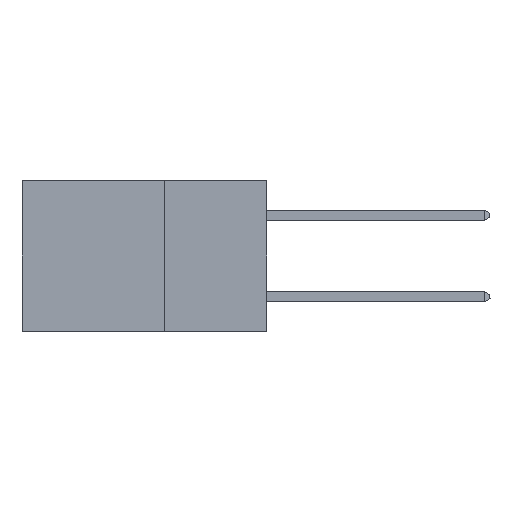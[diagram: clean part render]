
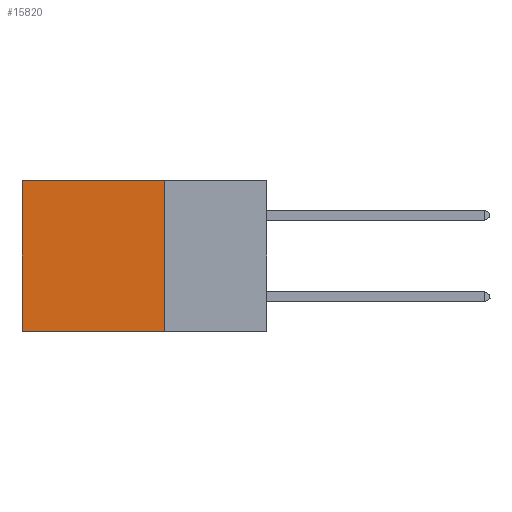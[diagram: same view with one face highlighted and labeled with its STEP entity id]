
A CAD part, left-side view. The second image highlights one B-rep face of the part: STEP entity #15820.
In plain terms, the highlighted planar face has unit normal (-1, 0, 0).
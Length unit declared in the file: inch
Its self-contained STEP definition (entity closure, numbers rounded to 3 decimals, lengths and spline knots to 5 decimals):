
#218 = ORIENTED_EDGE ( 'NONE', *, *, #1779, .F. ) ;
#876 = CARTESIAN_POINT ( 'NONE',  ( 0.2875, 0.6, 0. ) ) ;
#1040 = AXIS2_PLACEMENT_3D ( 'NONE', #15826, #5194, #15711 ) ;
#1613 = LINE ( 'NONE', #12355, #10148 ) ;
#1779 = EDGE_CURVE ( 'NONE', #7431, #14824, #11277, .T. ) ;
#2708 = FACE_OUTER_BOUND ( 'NONE', #6926, .T. ) ;
#3039 = ORIENTED_EDGE ( 'NONE', *, *, #9611, .F. ) ;
#3600 = CARTESIAN_POINT ( 'NONE',  ( 0.2875, 0.25, 0. ) ) ;
#4012 = LINE ( 'NONE', #876, #6762 ) ;
#4219 = EDGE_CURVE ( 'NONE', #12657, #14251, #1613, .T. ) ;
#5178 = ORIENTED_EDGE ( 'NONE', *, *, #13578, .T. ) ;
#5194 = DIRECTION ( 'NONE',  ( 1., 0., 0. ) ) ;
#5676 = CARTESIAN_POINT ( 'NONE',  ( 0.2875, 0.6, 0. ) ) ;
#6318 = ORIENTED_EDGE ( 'NONE', *, *, #4219, .T. ) ;
#6500 = VECTOR ( 'NONE', #16555, 39.37008 ) ;
#6762 = VECTOR ( 'NONE', #14345, 39.37008 ) ;
#6926 = EDGE_LOOP ( 'NONE', ( #5178, #218, #3039, #6318 ) ) ;
#7095 = CARTESIAN_POINT ( 'NONE',  ( 0.2875, 0.25, -0.37 ) ) ;
#7431 = VERTEX_POINT ( 'NONE', #8869 ) ;
#8869 = CARTESIAN_POINT ( 'NONE',  ( 0.2875, 0.25, -0.37 ) ) ;
#8874 = LINE ( 'NONE', #10557, #16418 ) ;
#9611 = EDGE_CURVE ( 'NONE', #12657, #7431, #8874, .T. ) ;
#10148 = VECTOR ( 'NONE', #13887, 39.37008 ) ;
#10557 = CARTESIAN_POINT ( 'NONE',  ( 0.2875, 0.25, 0. ) ) ;
#10917 = DIRECTION ( 'NONE',  ( 0., 0., -1. ) ) ;
#11277 = LINE ( 'NONE', #7095, #6500 ) ;
#12355 = CARTESIAN_POINT ( 'NONE',  ( 0.2875, 0.25, 0. ) ) ;
#12657 = VERTEX_POINT ( 'NONE', #3600 ) ;
#13190 = PLANE ( 'NONE',  #1040 ) ;
#13578 = EDGE_CURVE ( 'NONE', #14251, #14824, #4012, .T. ) ;
#13887 = DIRECTION ( 'NONE',  ( 0., 1., 0. ) ) ;
#14251 = VERTEX_POINT ( 'NONE', #5676 ) ;
#14345 = DIRECTION ( 'NONE',  ( 0., 0., -1. ) ) ;
#14824 = VERTEX_POINT ( 'NONE', #16892 ) ;
#15711 = DIRECTION ( 'NONE',  ( 0., 0., -1. ) ) ;
#15820 = ADVANCED_FACE ( 'NONE', ( #2708 ), #13190, .F. ) ;
#15826 = CARTESIAN_POINT ( 'NONE',  ( 0.2875, 0.25, 0. ) ) ;
#16418 = VECTOR ( 'NONE', #10917, 39.37008 ) ;
#16555 = DIRECTION ( 'NONE',  ( 0., 1., 0. ) ) ;
#16892 = CARTESIAN_POINT ( 'NONE',  ( 0.2875, 0.6, -0.37 ) ) ;
